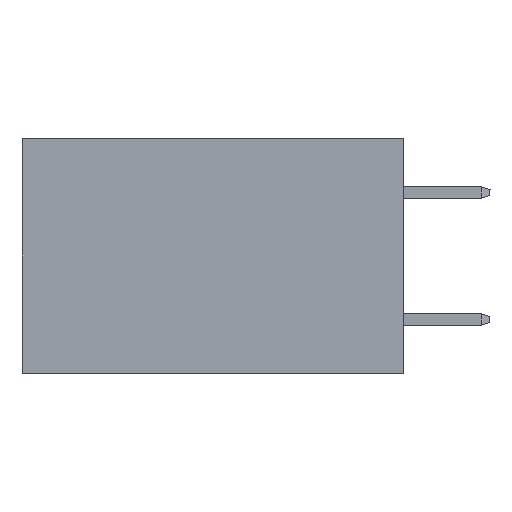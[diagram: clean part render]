
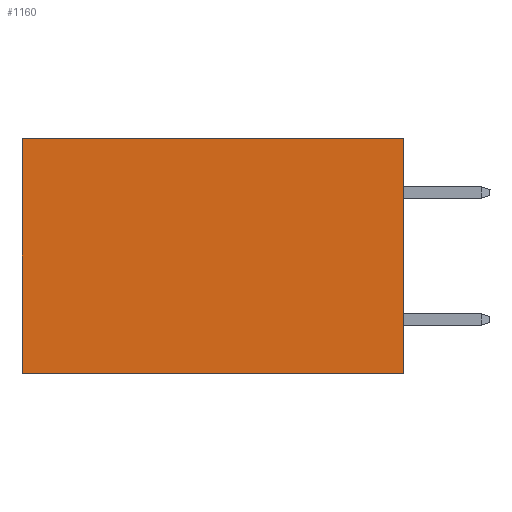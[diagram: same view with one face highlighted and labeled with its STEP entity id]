
A CAD part, left-side view. The second image highlights one B-rep face of the part: STEP entity #1160.
In plain terms, the highlighted planar face has unit normal (-1, 0, 0).
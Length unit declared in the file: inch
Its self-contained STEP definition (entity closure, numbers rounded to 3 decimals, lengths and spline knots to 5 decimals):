
#1016 = CARTESIAN_POINT ( 'NONE',  ( 0.2875, 0.6, 0. ) ) ;
#1160 = ADVANCED_FACE ( 'NONE', ( #17951 ), #17851, .F. ) ;
#2386 = LINE ( 'NONE', #16780, #8386 ) ;
#2566 = EDGE_CURVE ( 'NONE', #16182, #13505, #2386, .T. ) ;
#3259 = DIRECTION ( 'NONE',  ( 1., 0., 0. ) ) ;
#3339 = ORIENTED_EDGE ( 'NONE', *, *, #2566, .F. ) ;
#4185 = EDGE_LOOP ( 'NONE', ( #6855, #3339, #11461, #9820 ) ) ;
#4440 = DIRECTION ( 'NONE',  ( 0., 0., -1. ) ) ;
#4854 = VECTOR ( 'NONE', #4440, 39.37008 ) ;
#5673 = CARTESIAN_POINT ( 'NONE',  ( 0.2875, 0.6, 0. ) ) ;
#5960 = VERTEX_POINT ( 'NONE', #20170 ) ;
#6855 = ORIENTED_EDGE ( 'NONE', *, *, #10795, .T. ) ;
#7212 = DIRECTION ( 'NONE',  ( 0., 1., 0. ) ) ;
#8179 = CARTESIAN_POINT ( 'NONE',  ( 0.2875, 0., 0. ) ) ;
#8386 = VECTOR ( 'NONE', #7212, 39.37008 ) ;
#8530 = LINE ( 'NONE', #15015, #9309 ) ;
#9309 = VECTOR ( 'NONE', #16397, 39.37008 ) ;
#9761 = DIRECTION ( 'NONE',  ( 0., 0., -1. ) ) ;
#9820 = ORIENTED_EDGE ( 'NONE', *, *, #14350, .T. ) ;
#10384 = AXIS2_PLACEMENT_3D ( 'NONE', #8179, #3259, #9761 ) ;
#10795 = EDGE_CURVE ( 'NONE', #20548, #13505, #18615, .T. ) ;
#11461 = ORIENTED_EDGE ( 'NONE', *, *, #13679, .F. ) ;
#11670 = VECTOR ( 'NONE', #13829, 39.37008 ) ;
#13505 = VERTEX_POINT ( 'NONE', #18817 ) ;
#13679 = EDGE_CURVE ( 'NONE', #5960, #16182, #17326, .T. ) ;
#13829 = DIRECTION ( 'NONE',  ( 0., 0., -1. ) ) ;
#14239 = CARTESIAN_POINT ( 'NONE',  ( 0.2875, 0., 0. ) ) ;
#14350 = EDGE_CURVE ( 'NONE', #5960, #20548, #8530, .T. ) ;
#15015 = CARTESIAN_POINT ( 'NONE',  ( 0.2875, 0., 0. ) ) ;
#15339 = CARTESIAN_POINT ( 'NONE',  ( 0.2875, 0., -0.37 ) ) ;
#16182 = VERTEX_POINT ( 'NONE', #15339 ) ;
#16397 = DIRECTION ( 'NONE',  ( 0., 1., 0. ) ) ;
#16780 = CARTESIAN_POINT ( 'NONE',  ( 0.2875, 0., -0.37 ) ) ;
#17326 = LINE ( 'NONE', #14239, #4854 ) ;
#17851 = PLANE ( 'NONE',  #10384 ) ;
#17951 = FACE_OUTER_BOUND ( 'NONE', #4185, .T. ) ;
#18615 = LINE ( 'NONE', #1016, #11670 ) ;
#18817 = CARTESIAN_POINT ( 'NONE',  ( 0.2875, 0.6, -0.37 ) ) ;
#20170 = CARTESIAN_POINT ( 'NONE',  ( 0.2875, 0., 0. ) ) ;
#20548 = VERTEX_POINT ( 'NONE', #5673 ) ;
